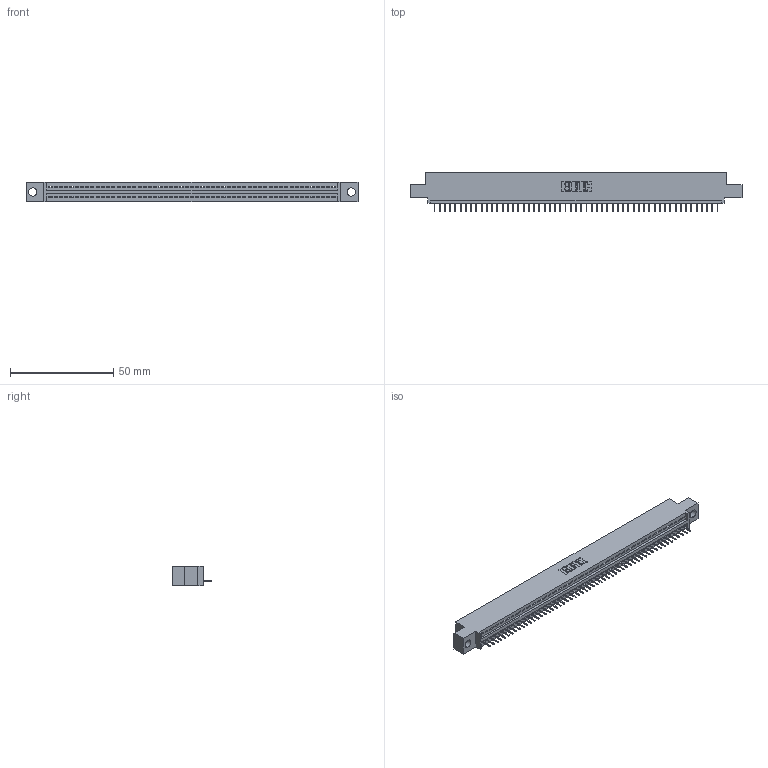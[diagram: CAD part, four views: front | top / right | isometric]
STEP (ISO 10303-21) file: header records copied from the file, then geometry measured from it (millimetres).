
FILE_DESCRIPTION (( 'STEP AP203' ), '1' );
FILE_NAME ('395-055-524-404.STEP', '2021-05-31T21:35:34', ( '' ), ( '' ), 'SwSTEP 2.0', 'SolidWorks 2020', '' );
FILE_SCHEMA (( 'CONFIG_CONTROL_DESIGN' ));
Length unit declared in the file: inch
Products named in the file (3): 345-292-001_345-293-124; 345 Part_0.110 Offset - 0.156 Dia-TI; 395-055-524-404
Assembly tree (56 placements, depth 2):
  395-055-524-404
    345 Part_0.110 Offset - 0.156 Dia-TI
    345-292-001_345-293-124  x55
Bounding box: 160.91 x 19.35 x 9.4 mm (x, y, z)
Volume: 14993.2 mm3; surface area: 19331 mm2
Topology: 56 solids, 56 shells, 3554 faces, 10289 edges, 6638 vertices
Faces by surface type: plane 2628, cylinder 926
Entity records: 40269 total; most frequent: CARTESIAN_POINT 6983, ORIENTED_EDGE 6970, DIRECTION 6079, EDGE_CURVE 3485, VECTOR 3137, LINE 3137, VERTEX_POINT 2318, AXIS2_PLACEMENT_3D 1471
